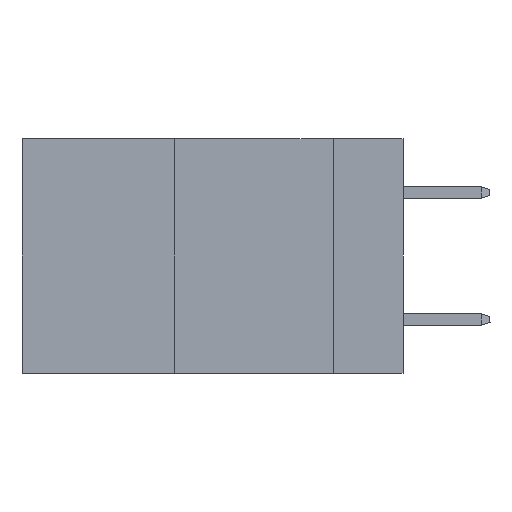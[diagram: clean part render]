
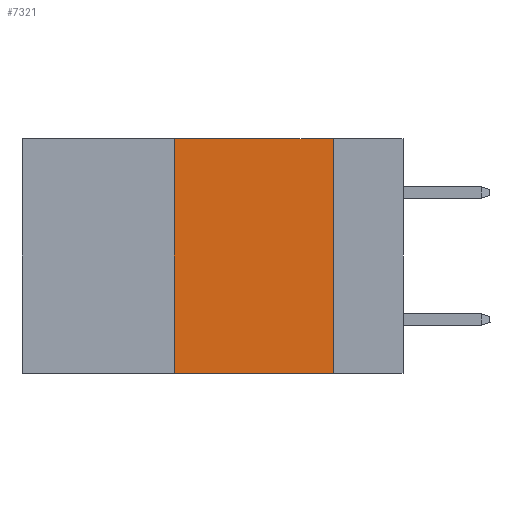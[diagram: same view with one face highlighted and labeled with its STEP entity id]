
A CAD part, left-side view. The second image highlights one B-rep face of the part: STEP entity #7321.
In plain terms, the highlighted planar face has unit normal (-1, 0, 0).
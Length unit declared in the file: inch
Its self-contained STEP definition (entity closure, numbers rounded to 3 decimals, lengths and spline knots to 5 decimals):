
#107 = EDGE_CURVE ( 'NONE', #7515, #425, #6053, .T. ) ;
#181 = FACE_OUTER_BOUND ( 'NONE', #4752, .T. ) ;
#251 = DIRECTION ( 'NONE',  ( 0., 0., -1. ) ) ;
#425 = VERTEX_POINT ( 'NONE', #10444 ) ;
#1086 = ORIENTED_EDGE ( 'NONE', *, *, #107, .F. ) ;
#1235 = CARTESIAN_POINT ( 'NONE',  ( 0., 0.36, -0.37 ) ) ;
#1981 = DIRECTION ( 'NONE',  ( 0., 0., 1. ) ) ;
#2276 = DIRECTION ( 'NONE',  ( 0., 0., -1. ) ) ;
#2410 = CARTESIAN_POINT ( 'NONE',  ( 0., 0.11, 0. ) ) ;
#2579 = LINE ( 'NONE', #3680, #11326 ) ;
#3465 = ORIENTED_EDGE ( 'NONE', *, *, #12261, .T. ) ;
#3680 = CARTESIAN_POINT ( 'NONE',  ( 0., 0.6, 0. ) ) ;
#3990 = CARTESIAN_POINT ( 'NONE',  ( 0., 0.11, 0. ) ) ;
#4073 = DIRECTION ( 'NONE',  ( 1., 0., 0. ) ) ;
#4752 = EDGE_LOOP ( 'NONE', ( #1086, #10258, #10858, #3465 ) ) ;
#5904 = PLANE ( 'NONE',  #9917 ) ;
#6053 = LINE ( 'NONE', #3990, #9931 ) ;
#6249 = CARTESIAN_POINT ( 'NONE',  ( 0., 0.6, -0.37 ) ) ;
#6317 = LINE ( 'NONE', #6249, #8119 ) ;
#6402 = VERTEX_POINT ( 'NONE', #9623 ) ;
#6868 = VERTEX_POINT ( 'NONE', #1235 ) ;
#6911 = CARTESIAN_POINT ( 'NONE',  ( 0., 0.6, 0. ) ) ;
#7321 = ADVANCED_FACE ( 'NONE', ( #181 ), #5904, .F. ) ;
#7515 = VERTEX_POINT ( 'NONE', #2410 ) ;
#7623 = DIRECTION ( 'NONE',  ( 0., -1., 0. ) ) ;
#8119 = VECTOR ( 'NONE', #7623, 39.37008 ) ;
#9352 = DIRECTION ( 'NONE',  ( 0., -1., 0. ) ) ;
#9623 = CARTESIAN_POINT ( 'NONE',  ( 0., 0.36, 0. ) ) ;
#9682 = LINE ( 'NONE', #10576, #11913 ) ;
#9917 = AXIS2_PLACEMENT_3D ( 'NONE', #6911, #4073, #2276 ) ;
#9931 = VECTOR ( 'NONE', #251, 39.37008 ) ;
#10258 = ORIENTED_EDGE ( 'NONE', *, *, #11802, .F. ) ;
#10444 = CARTESIAN_POINT ( 'NONE',  ( 0., 0.11, -0.37 ) ) ;
#10576 = CARTESIAN_POINT ( 'NONE',  ( 0., 0.36, 0. ) ) ;
#10858 = ORIENTED_EDGE ( 'NONE', *, *, #11185, .F. ) ;
#11185 = EDGE_CURVE ( 'NONE', #6868, #6402, #9682, .T. ) ;
#11326 = VECTOR ( 'NONE', #9352, 39.37008 ) ;
#11802 = EDGE_CURVE ( 'NONE', #6402, #7515, #2579, .T. ) ;
#11913 = VECTOR ( 'NONE', #1981, 39.37008 ) ;
#12261 = EDGE_CURVE ( 'NONE', #6868, #425, #6317, .T. ) ;
